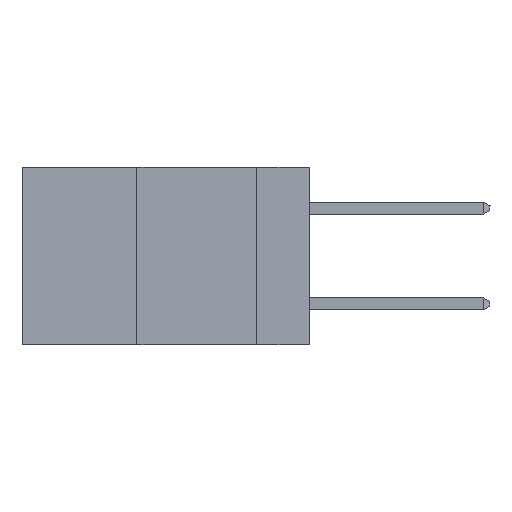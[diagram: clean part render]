
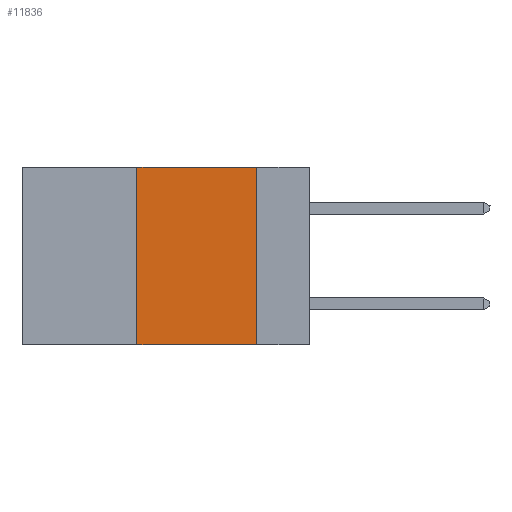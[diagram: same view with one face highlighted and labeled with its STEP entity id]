
A CAD part, left-side view. The second image highlights one B-rep face of the part: STEP entity #11836.
In plain terms, the highlighted planar face has unit normal (-1, 0, 0).
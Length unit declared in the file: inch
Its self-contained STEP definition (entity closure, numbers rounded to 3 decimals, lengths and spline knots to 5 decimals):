
#133 = VECTOR ( 'NONE', #17893, 39.37008 ) ;
#648 = CARTESIAN_POINT ( 'NONE',  ( 0., 0.6, 0. ) ) ;
#878 = CARTESIAN_POINT ( 'NONE',  ( 0., 0.11, -0.37 ) ) ;
#999 = VECTOR ( 'NONE', #14867, 39.37008 ) ;
#1204 = DIRECTION ( 'NONE',  ( 0., 0., -1. ) ) ;
#1350 = VERTEX_POINT ( 'NONE', #37752 ) ;
#2015 = AXIS2_PLACEMENT_3D ( 'NONE', #648, #3805, #25228 ) ;
#2258 = FACE_OUTER_BOUND ( 'NONE', #32020, .T. ) ;
#3805 = DIRECTION ( 'NONE',  ( 1., 0., 0. ) ) ;
#4266 = ORIENTED_EDGE ( 'NONE', *, *, #15043, .F. ) ;
#6507 = LINE ( 'NONE', #37477, #13714 ) ;
#8698 = VERTEX_POINT ( 'NONE', #22591 ) ;
#10389 = CARTESIAN_POINT ( 'NONE',  ( 0., 0.11, 0. ) ) ;
#11156 = VERTEX_POINT ( 'NONE', #27533 ) ;
#11836 = ADVANCED_FACE ( 'NONE', ( #2258 ), #22217, .F. ) ;
#13202 = DIRECTION ( 'NONE',  ( 0., 0., 1. ) ) ;
#13714 = VECTOR ( 'NONE', #13202, 39.37008 ) ;
#14867 = DIRECTION ( 'NONE',  ( 0., -1., 0. ) ) ;
#15043 = EDGE_CURVE ( 'NONE', #11156, #25369, #25517, .T. ) ;
#15851 = ORIENTED_EDGE ( 'NONE', *, *, #23750, .T. ) ;
#17893 = DIRECTION ( 'NONE',  ( 0., -1., 0. ) ) ;
#20343 = LINE ( 'NONE', #33073, #999 ) ;
#20860 = ORIENTED_EDGE ( 'NONE', *, *, #36635, .F. ) ;
#22217 = PLANE ( 'NONE',  #2015 ) ;
#22591 = CARTESIAN_POINT ( 'NONE',  ( 0., 0.36, -0.37 ) ) ;
#23750 = EDGE_CURVE ( 'NONE', #8698, #25369, #31782, .T. ) ;
#24587 = VECTOR ( 'NONE', #1204, 39.37008 ) ;
#25228 = DIRECTION ( 'NONE',  ( 0., 0., -1. ) ) ;
#25369 = VERTEX_POINT ( 'NONE', #878 ) ;
#25517 = LINE ( 'NONE', #10389, #24587 ) ;
#27533 = CARTESIAN_POINT ( 'NONE',  ( 0., 0.11, 0. ) ) ;
#27658 = ORIENTED_EDGE ( 'NONE', *, *, #38273, .F. ) ;
#31782 = LINE ( 'NONE', #35972, #133 ) ;
#32020 = EDGE_LOOP ( 'NONE', ( #4266, #27658, #20860, #15851 ) ) ;
#33073 = CARTESIAN_POINT ( 'NONE',  ( 0., 0.6, 0. ) ) ;
#35972 = CARTESIAN_POINT ( 'NONE',  ( 0., 0.6, -0.37 ) ) ;
#36635 = EDGE_CURVE ( 'NONE', #8698, #1350, #6507, .T. ) ;
#37477 = CARTESIAN_POINT ( 'NONE',  ( 0., 0.36, 0. ) ) ;
#37752 = CARTESIAN_POINT ( 'NONE',  ( 0., 0.36, 0. ) ) ;
#38273 = EDGE_CURVE ( 'NONE', #1350, #11156, #20343, .T. ) ;
